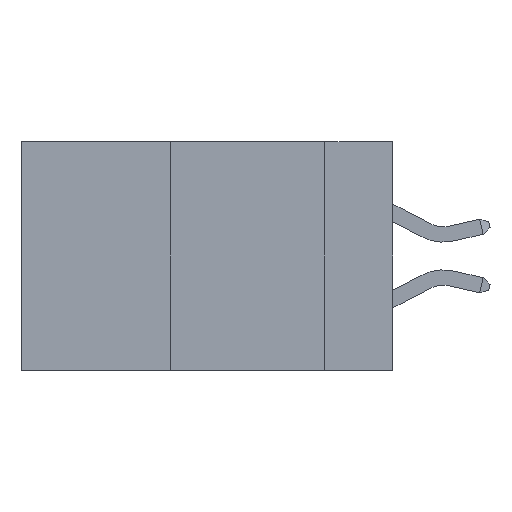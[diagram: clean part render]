
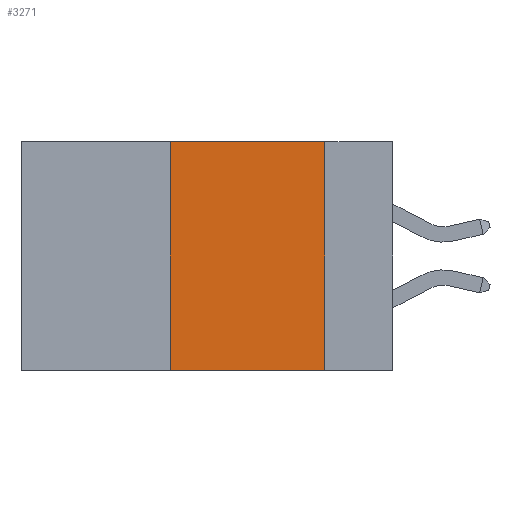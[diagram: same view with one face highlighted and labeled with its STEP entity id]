
A CAD part, left-side view. The second image highlights one B-rep face of the part: STEP entity #3271.
In plain terms, the highlighted planar face has unit normal (-1, 0, 0).
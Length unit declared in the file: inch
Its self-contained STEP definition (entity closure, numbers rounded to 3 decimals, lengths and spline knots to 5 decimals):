
#359 = DIRECTION ( 'NONE',  ( 0., -1., 0. ) ) ;
#955 = CARTESIAN_POINT ( 'NONE',  ( 0., 0.36, 0. ) ) ;
#1419 = CARTESIAN_POINT ( 'NONE',  ( 0., 0.36, 0. ) ) ;
#3271 = ADVANCED_FACE ( 'NONE', ( #13184 ), #8962, .F. ) ;
#3295 = CARTESIAN_POINT ( 'NONE',  ( 0., 0.6, 0. ) ) ;
#3740 = VERTEX_POINT ( 'NONE', #9865 ) ;
#4784 = VERTEX_POINT ( 'NONE', #9542 ) ;
#5222 = VECTOR ( 'NONE', #10680, 39.37008 ) ;
#5784 = LINE ( 'NONE', #1419, #20749 ) ;
#6513 = VECTOR ( 'NONE', #359, 39.37008 ) ;
#6858 = DIRECTION ( 'NONE',  ( 0., 0., -1. ) ) ;
#7148 = ORIENTED_EDGE ( 'NONE', *, *, #13110, .F. ) ;
#7334 = DIRECTION ( 'NONE',  ( 0., 0., -1. ) ) ;
#8962 = PLANE ( 'NONE',  #23451 ) ;
#9535 = LINE ( 'NONE', #18234, #18525 ) ;
#9542 = CARTESIAN_POINT ( 'NONE',  ( 0., 0.36, -0.37 ) ) ;
#9865 = CARTESIAN_POINT ( 'NONE',  ( 0., 0.11, 0. ) ) ;
#10558 = VERTEX_POINT ( 'NONE', #955 ) ;
#10680 = DIRECTION ( 'NONE',  ( 0., -1., 0. ) ) ;
#11741 = EDGE_CURVE ( 'NONE', #10558, #3740, #16077, .T. ) ;
#12238 = ORIENTED_EDGE ( 'NONE', *, *, #11741, .F. ) ;
#12434 = ORIENTED_EDGE ( 'NONE', *, *, #17010, .F. ) ;
#12595 = CARTESIAN_POINT ( 'NONE',  ( 0., 0.6, 0. ) ) ;
#13110 = EDGE_CURVE ( 'NONE', #3740, #20029, #9535, .T. ) ;
#13184 = FACE_OUTER_BOUND ( 'NONE', #22363, .T. ) ;
#14398 = DIRECTION ( 'NONE',  ( 1., 0., 0. ) ) ;
#15864 = CARTESIAN_POINT ( 'NONE',  ( 0., 0.11, -0.37 ) ) ;
#16016 = DIRECTION ( 'NONE',  ( 0., 0., 1. ) ) ;
#16077 = LINE ( 'NONE', #12595, #6513 ) ;
#16711 = ORIENTED_EDGE ( 'NONE', *, *, #17124, .T. ) ;
#17010 = EDGE_CURVE ( 'NONE', #4784, #10558, #5784, .T. ) ;
#17124 = EDGE_CURVE ( 'NONE', #4784, #20029, #20176, .T. ) ;
#18234 = CARTESIAN_POINT ( 'NONE',  ( 0., 0.11, 0. ) ) ;
#18525 = VECTOR ( 'NONE', #7334, 39.37008 ) ;
#20029 = VERTEX_POINT ( 'NONE', #15864 ) ;
#20176 = LINE ( 'NONE', #21646, #5222 ) ;
#20749 = VECTOR ( 'NONE', #16016, 39.37008 ) ;
#21646 = CARTESIAN_POINT ( 'NONE',  ( 0., 0.6, -0.37 ) ) ;
#22363 = EDGE_LOOP ( 'NONE', ( #7148, #12238, #12434, #16711 ) ) ;
#23451 = AXIS2_PLACEMENT_3D ( 'NONE', #3295, #14398, #6858 ) ;
